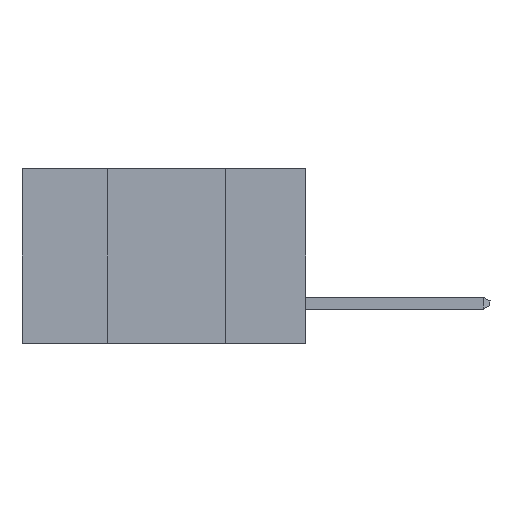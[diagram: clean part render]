
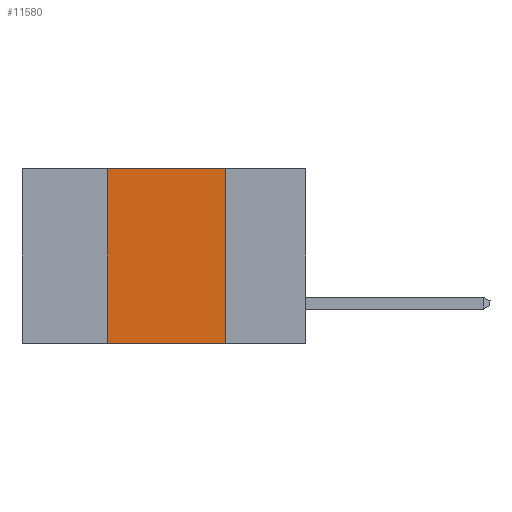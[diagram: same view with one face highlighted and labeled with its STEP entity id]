
A CAD part, left-side view. The second image highlights one B-rep face of the part: STEP entity #11580.
In plain terms, the highlighted planar face has unit normal (-1, 0, 0).
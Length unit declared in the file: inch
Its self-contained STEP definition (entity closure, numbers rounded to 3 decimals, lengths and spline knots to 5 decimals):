
#151 = CARTESIAN_POINT ( 'NONE',  ( 0., 0.6, 0. ) ) ;
#413 = ORIENTED_EDGE ( 'NONE', *, *, #7914, .F. ) ;
#788 = DIRECTION ( 'NONE',  ( 0., 0., 1. ) ) ;
#1370 = LINE ( 'NONE', #7722, #19303 ) ;
#1385 = VECTOR ( 'NONE', #13135, 39.37008 ) ;
#2748 = VECTOR ( 'NONE', #14698, 39.37008 ) ;
#3303 = ORIENTED_EDGE ( 'NONE', *, *, #8709, .F. ) ;
#3974 = ORIENTED_EDGE ( 'NONE', *, *, #8706, .T. ) ;
#5462 = LINE ( 'NONE', #16162, #2748 ) ;
#5829 = CARTESIAN_POINT ( 'NONE',  ( 0., 0.6, 0. ) ) ;
#6375 = EDGE_CURVE ( 'NONE', #9016, #11728, #8147, .T. ) ;
#6539 = ORIENTED_EDGE ( 'NONE', *, *, #6375, .F. ) ;
#6599 = CARTESIAN_POINT ( 'NONE',  ( 0., 0.17, -0.37 ) ) ;
#7722 = CARTESIAN_POINT ( 'NONE',  ( 0., 0.42, -0.37 ) ) ;
#7914 = EDGE_CURVE ( 'NONE', #10597, #9016, #1370, .T. ) ;
#8147 = LINE ( 'NONE', #151, #15600 ) ;
#8264 = LINE ( 'NONE', #14595, #1385 ) ;
#8706 = EDGE_CURVE ( 'NONE', #10597, #16535, #5462, .T. ) ;
#8709 = EDGE_CURVE ( 'NONE', #11728, #16535, #8264, .T. ) ;
#8888 = CARTESIAN_POINT ( 'NONE',  ( 0., 0.42, -0.37 ) ) ;
#9016 = VERTEX_POINT ( 'NONE', #14190 ) ;
#9133 = DIRECTION ( 'NONE',  ( 1., 0., 0. ) ) ;
#10008 = EDGE_LOOP ( 'NONE', ( #3303, #6539, #413, #3974 ) ) ;
#10597 = VERTEX_POINT ( 'NONE', #8888 ) ;
#11580 = ADVANCED_FACE ( 'NONE', ( #15271 ), #15581, .F. ) ;
#11728 = VERTEX_POINT ( 'NONE', #15479 ) ;
#12514 = DIRECTION ( 'NONE',  ( 0., -1., 0. ) ) ;
#13135 = DIRECTION ( 'NONE',  ( 0., 0., -1. ) ) ;
#13916 = DIRECTION ( 'NONE',  ( 0., 0., -1. ) ) ;
#14190 = CARTESIAN_POINT ( 'NONE',  ( 0., 0.42, 0. ) ) ;
#14595 = CARTESIAN_POINT ( 'NONE',  ( 0., 0.17, -0.37 ) ) ;
#14698 = DIRECTION ( 'NONE',  ( 0., -1., 0. ) ) ;
#15271 = FACE_OUTER_BOUND ( 'NONE', #10008, .T. ) ;
#15372 = AXIS2_PLACEMENT_3D ( 'NONE', #5829, #9133, #13916 ) ;
#15479 = CARTESIAN_POINT ( 'NONE',  ( 0., 0.17, 0. ) ) ;
#15581 = PLANE ( 'NONE',  #15372 ) ;
#15600 = VECTOR ( 'NONE', #12514, 39.37008 ) ;
#16162 = CARTESIAN_POINT ( 'NONE',  ( 0., 0.6, -0.37 ) ) ;
#16535 = VERTEX_POINT ( 'NONE', #6599 ) ;
#19303 = VECTOR ( 'NONE', #788, 39.37008 ) ;
